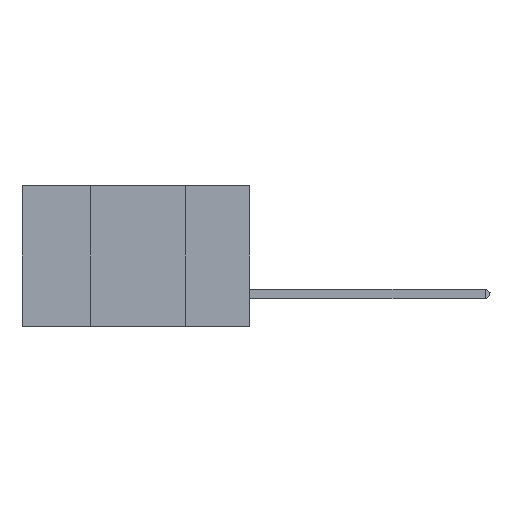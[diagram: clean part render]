
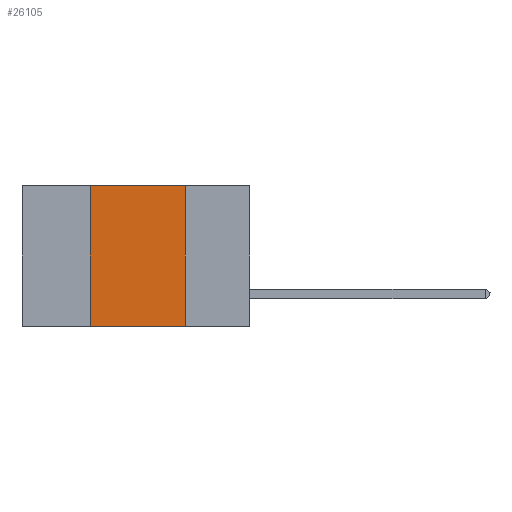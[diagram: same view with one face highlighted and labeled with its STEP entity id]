
A CAD part, left-side view. The second image highlights one B-rep face of the part: STEP entity #26105.
In plain terms, the highlighted planar face has unit normal (-1, 0, 0).
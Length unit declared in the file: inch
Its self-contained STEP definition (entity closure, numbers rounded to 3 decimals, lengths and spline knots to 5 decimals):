
#105 = CARTESIAN_POINT ( 'NONE',  ( 0., 0.17, 0. ) ) ;
#371 = ORIENTED_EDGE ( 'NONE', *, *, #9573, .F. ) ;
#1668 = LINE ( 'NONE', #4517, #7662 ) ;
#4517 = CARTESIAN_POINT ( 'NONE',  ( 0., 0.6, 0. ) ) ;
#5365 = ORIENTED_EDGE ( 'NONE', *, *, #30195, .T. ) ;
#5830 = EDGE_CURVE ( 'NONE', #20899, #29217, #1668, .T. ) ;
#7662 = VECTOR ( 'NONE', #28708, 39.37008 ) ;
#7742 = CARTESIAN_POINT ( 'NONE',  ( 0., 0.6, 0. ) ) ;
#9358 = CARTESIAN_POINT ( 'NONE',  ( 0., 0.6, -0.37 ) ) ;
#9573 = EDGE_CURVE ( 'NONE', #29217, #20989, #42341, .T. ) ;
#11877 = ORIENTED_EDGE ( 'NONE', *, *, #12655, .F. ) ;
#12655 = EDGE_CURVE ( 'NONE', #31824, #20899, #17531, .T. ) ;
#13230 = DIRECTION ( 'NONE',  ( 0., 0., -1. ) ) ;
#14463 = CARTESIAN_POINT ( 'NONE',  ( 0., 0.42, 0. ) ) ;
#14838 = VECTOR ( 'NONE', #13230, 39.37008 ) ;
#15039 = EDGE_LOOP ( 'NONE', ( #371, #36266, #11877, #5365 ) ) ;
#16360 = DIRECTION ( 'NONE',  ( 0., -1., 0. ) ) ;
#16757 = VECTOR ( 'NONE', #16360, 39.37008 ) ;
#17531 = LINE ( 'NONE', #14463, #34708 ) ;
#18650 = CARTESIAN_POINT ( 'NONE',  ( 0., 0.42, -0.37 ) ) ;
#19862 = DIRECTION ( 'NONE',  ( 0., 0., -1. ) ) ;
#20899 = VERTEX_POINT ( 'NONE', #26433 ) ;
#20989 = VERTEX_POINT ( 'NONE', #28544 ) ;
#21384 = CARTESIAN_POINT ( 'NONE',  ( 0., 0.17, 0. ) ) ;
#23265 = AXIS2_PLACEMENT_3D ( 'NONE', #7742, #37340, #19862 ) ;
#23324 = LINE ( 'NONE', #9358, #16757 ) ;
#26105 = ADVANCED_FACE ( 'NONE', ( #32494 ), #36189, .F. ) ;
#26433 = CARTESIAN_POINT ( 'NONE',  ( 0., 0.42, 0. ) ) ;
#28544 = CARTESIAN_POINT ( 'NONE',  ( 0., 0.17, -0.37 ) ) ;
#28708 = DIRECTION ( 'NONE',  ( 0., -1., 0. ) ) ;
#29217 = VERTEX_POINT ( 'NONE', #21384 ) ;
#30195 = EDGE_CURVE ( 'NONE', #31824, #20989, #23324, .T. ) ;
#31824 = VERTEX_POINT ( 'NONE', #18650 ) ;
#32494 = FACE_OUTER_BOUND ( 'NONE', #15039, .T. ) ;
#34708 = VECTOR ( 'NONE', #41373, 39.37008 ) ;
#36189 = PLANE ( 'NONE',  #23265 ) ;
#36266 = ORIENTED_EDGE ( 'NONE', *, *, #5830, .F. ) ;
#37340 = DIRECTION ( 'NONE',  ( 1., 0., 0. ) ) ;
#41373 = DIRECTION ( 'NONE',  ( 0., 0., 1. ) ) ;
#42341 = LINE ( 'NONE', #105, #14838 ) ;
